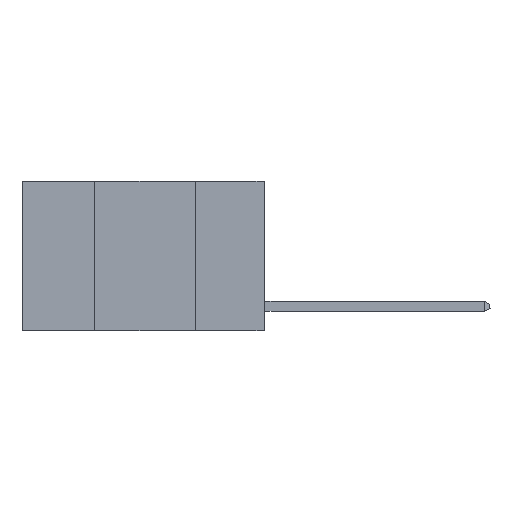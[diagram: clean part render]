
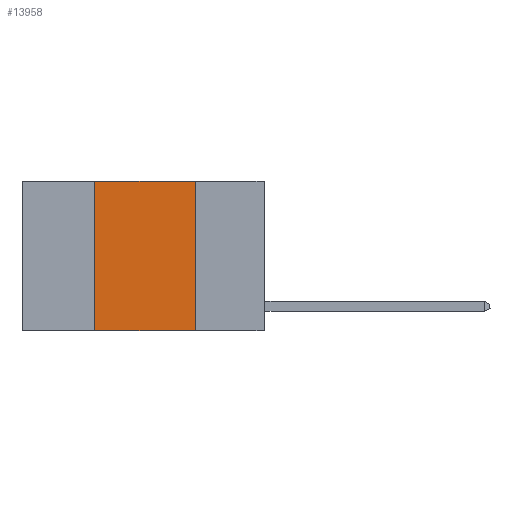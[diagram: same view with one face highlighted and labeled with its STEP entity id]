
A CAD part, left-side view. The second image highlights one B-rep face of the part: STEP entity #13958.
In plain terms, the highlighted planar face has unit normal (-1, 0, 0).
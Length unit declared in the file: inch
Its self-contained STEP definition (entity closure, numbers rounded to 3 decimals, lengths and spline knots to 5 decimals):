
#214 = LINE ( 'NONE', #15281, #7247 ) ;
#319 = VECTOR ( 'NONE', #15058, 39.37008 ) ;
#1100 = VECTOR ( 'NONE', #6639, 39.37008 ) ;
#1148 = DIRECTION ( 'NONE',  ( 0., 0., 1. ) ) ;
#1585 = CARTESIAN_POINT ( 'NONE',  ( 0., 0.6, 0. ) ) ;
#1704 = CARTESIAN_POINT ( 'NONE',  ( 0., 0.17, -0.37 ) ) ;
#2244 = EDGE_CURVE ( 'NONE', #10059, #9216, #214, .T. ) ;
#3655 = CARTESIAN_POINT ( 'NONE',  ( 0., 0.6, 0. ) ) ;
#4292 = ORIENTED_EDGE ( 'NONE', *, *, #10097, .F. ) ;
#4882 = VERTEX_POINT ( 'NONE', #1704 ) ;
#5286 = CARTESIAN_POINT ( 'NONE',  ( 0., 0.17, 0. ) ) ;
#5339 = AXIS2_PLACEMENT_3D ( 'NONE', #3655, #15179, #7605 ) ;
#5730 = ORIENTED_EDGE ( 'NONE', *, *, #6951, .T. ) ;
#5774 = LINE ( 'NONE', #8338, #319 ) ;
#6639 = DIRECTION ( 'NONE',  ( 0., -1., 0. ) ) ;
#6951 = EDGE_CURVE ( 'NONE', #10059, #4882, #5774, .T. ) ;
#7132 = VECTOR ( 'NONE', #14328, 39.37008 ) ;
#7247 = VECTOR ( 'NONE', #1148, 39.37008 ) ;
#7605 = DIRECTION ( 'NONE',  ( 0., 0., -1. ) ) ;
#7899 = LINE ( 'NONE', #1585, #1100 ) ;
#7927 = VERTEX_POINT ( 'NONE', #13588 ) ;
#8041 = ORIENTED_EDGE ( 'NONE', *, *, #2244, .F. ) ;
#8097 = LINE ( 'NONE', #5286, #7132 ) ;
#8338 = CARTESIAN_POINT ( 'NONE',  ( 0., 0.6, -0.37 ) ) ;
#8579 = ORIENTED_EDGE ( 'NONE', *, *, #10955, .F. ) ;
#9004 = FACE_OUTER_BOUND ( 'NONE', #14782, .T. ) ;
#9097 = CARTESIAN_POINT ( 'NONE',  ( 0., 0.42, -0.37 ) ) ;
#9216 = VERTEX_POINT ( 'NONE', #16336 ) ;
#10059 = VERTEX_POINT ( 'NONE', #9097 ) ;
#10097 = EDGE_CURVE ( 'NONE', #7927, #4882, #8097, .T. ) ;
#10955 = EDGE_CURVE ( 'NONE', #9216, #7927, #7899, .T. ) ;
#13588 = CARTESIAN_POINT ( 'NONE',  ( 0., 0.17, 0. ) ) ;
#13958 = ADVANCED_FACE ( 'NONE', ( #9004 ), #15343, .F. ) ;
#14328 = DIRECTION ( 'NONE',  ( 0., 0., -1. ) ) ;
#14782 = EDGE_LOOP ( 'NONE', ( #4292, #8579, #8041, #5730 ) ) ;
#15058 = DIRECTION ( 'NONE',  ( 0., -1., 0. ) ) ;
#15179 = DIRECTION ( 'NONE',  ( 1., 0., 0. ) ) ;
#15281 = CARTESIAN_POINT ( 'NONE',  ( 0., 0.42, 0. ) ) ;
#15343 = PLANE ( 'NONE',  #5339 ) ;
#16336 = CARTESIAN_POINT ( 'NONE',  ( 0., 0.42, 0. ) ) ;
